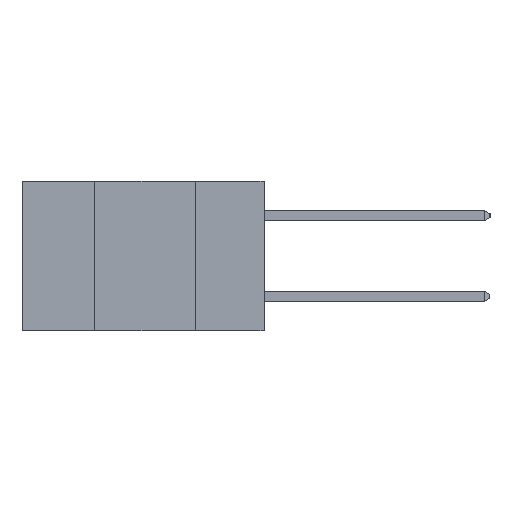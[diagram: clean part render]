
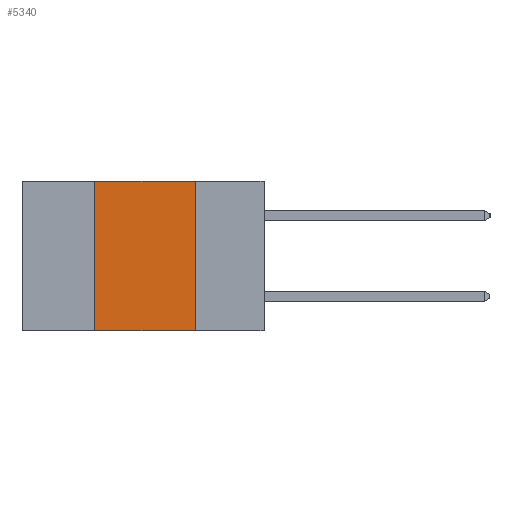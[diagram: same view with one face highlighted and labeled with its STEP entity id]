
A CAD part, left-side view. The second image highlights one B-rep face of the part: STEP entity #5340.
In plain terms, the highlighted planar face has unit normal (-1, 0, 0).
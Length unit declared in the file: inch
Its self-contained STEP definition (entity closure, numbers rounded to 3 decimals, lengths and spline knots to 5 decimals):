
#1603 = DIRECTION ( 'NONE',  ( 0., 0., -1. ) ) ;
#1627 = DIRECTION ( 'NONE',  ( 1., 0., 0. ) ) ;
#1652 = CARTESIAN_POINT ( 'NONE',  ( 0., 0.6, 0. ) ) ;
#1699 = CARTESIAN_POINT ( 'NONE',  ( 0., 0.6, 0. ) ) ;
#1752 = PLANE ( 'NONE',  #21625 ) ;
#1930 = FACE_OUTER_BOUND ( 'NONE', #19327, .T. ) ;
#3525 = VECTOR ( 'NONE', #10897, 39.37008 ) ;
#3594 = DIRECTION ( 'NONE',  ( 0., -1., 0. ) ) ;
#5340 = ADVANCED_FACE ( 'NONE', ( #1930 ), #1752, .F. ) ;
#7369 = DIRECTION ( 'NONE',  ( 0., -1., 0. ) ) ;
#7991 = CARTESIAN_POINT ( 'NONE',  ( 0., 0.17, 0. ) ) ;
#10044 = VERTEX_POINT ( 'NONE', #20847 ) ;
#10424 = EDGE_CURVE ( 'NONE', #20287, #10527, #15078, .T. ) ;
#10527 = VERTEX_POINT ( 'NONE', #22144 ) ;
#10795 = VECTOR ( 'NONE', #7369, 39.37008 ) ;
#10897 = DIRECTION ( 'NONE',  ( 0., 0., 1. ) ) ;
#11267 = VERTEX_POINT ( 'NONE', #7991 ) ;
#11618 = VECTOR ( 'NONE', #22345, 39.37008 ) ;
#11668 = EDGE_CURVE ( 'NONE', #20287, #10044, #22991, .T. ) ;
#13530 = LINE ( 'NONE', #1699, #17775 ) ;
#14125 = EDGE_CURVE ( 'NONE', #10044, #11267, #13530, .T. ) ;
#14737 = ORIENTED_EDGE ( 'NONE', *, *, #16521, .F. ) ;
#15078 = LINE ( 'NONE', #18355, #10795 ) ;
#15228 = ORIENTED_EDGE ( 'NONE', *, *, #10424, .T. ) ;
#15484 = ORIENTED_EDGE ( 'NONE', *, *, #11668, .F. ) ;
#16366 = ORIENTED_EDGE ( 'NONE', *, *, #14125, .F. ) ;
#16521 = EDGE_CURVE ( 'NONE', #11267, #10527, #17598, .T. ) ;
#17598 = LINE ( 'NONE', #20550, #11618 ) ;
#17775 = VECTOR ( 'NONE', #3594, 39.37008 ) ;
#18355 = CARTESIAN_POINT ( 'NONE',  ( 0., 0.6, -0.37 ) ) ;
#19327 = EDGE_LOOP ( 'NONE', ( #14737, #16366, #15484, #15228 ) ) ;
#19585 = CARTESIAN_POINT ( 'NONE',  ( 0., 0.42, -0.37 ) ) ;
#19983 = CARTESIAN_POINT ( 'NONE',  ( 0., 0.42, -0.37 ) ) ;
#20287 = VERTEX_POINT ( 'NONE', #19585 ) ;
#20550 = CARTESIAN_POINT ( 'NONE',  ( 0., 0.17, -0.37 ) ) ;
#20847 = CARTESIAN_POINT ( 'NONE',  ( 0., 0.42, 0. ) ) ;
#21625 = AXIS2_PLACEMENT_3D ( 'NONE', #1652, #1627, #1603 ) ;
#22144 = CARTESIAN_POINT ( 'NONE',  ( 0., 0.17, -0.37 ) ) ;
#22345 = DIRECTION ( 'NONE',  ( 0., 0., -1. ) ) ;
#22991 = LINE ( 'NONE', #19983, #3525 ) ;
